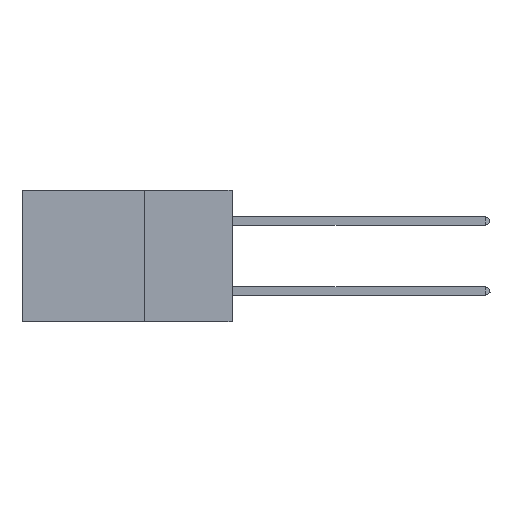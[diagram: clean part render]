
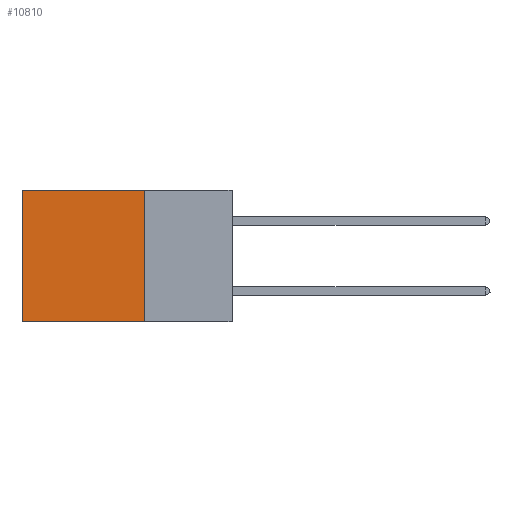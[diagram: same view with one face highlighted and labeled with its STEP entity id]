
A CAD part, left-side view. The second image highlights one B-rep face of the part: STEP entity #10810.
In plain terms, the highlighted planar face has unit normal (-1, 0, 0).
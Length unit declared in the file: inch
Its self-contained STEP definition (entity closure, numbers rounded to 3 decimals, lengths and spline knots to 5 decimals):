
#69 = VECTOR ( 'NONE', #7618, 39.37008 ) ;
#397 = DIRECTION ( 'NONE',  ( 0., 0., -1. ) ) ;
#1990 = DIRECTION ( 'NONE',  ( 0., 0., -1. ) ) ;
#3518 = VECTOR ( 'NONE', #1990, 39.37008 ) ;
#4175 = ORIENTED_EDGE ( 'NONE', *, *, #9058, .T. ) ;
#5876 = LINE ( 'NONE', #9888, #69 ) ;
#6025 = CARTESIAN_POINT ( 'NONE',  ( 0.2875, 0.25, -0.375 ) ) ;
#6129 = CARTESIAN_POINT ( 'NONE',  ( 0.2875, 0.6, -0.375 ) ) ;
#6674 = CARTESIAN_POINT ( 'NONE',  ( 0.2875, 0.25, -0.375 ) ) ;
#6875 = VERTEX_POINT ( 'NONE', #7212 ) ;
#6950 = VECTOR ( 'NONE', #9644, 39.37008 ) ;
#7188 = EDGE_CURVE ( 'NONE', #10684, #15488, #7501, .T. ) ;
#7212 = CARTESIAN_POINT ( 'NONE',  ( 0.2875, 0.6, -0.375 ) ) ;
#7288 = CARTESIAN_POINT ( 'NONE',  ( 0.2875, 0.25, 0. ) ) ;
#7501 = LINE ( 'NONE', #6674, #3518 ) ;
#7618 = DIRECTION ( 'NONE',  ( 0., 1., 0. ) ) ;
#7906 = EDGE_CURVE ( 'NONE', #11534, #6875, #13847, .T. ) ;
#9058 = EDGE_CURVE ( 'NONE', #10684, #11534, #11469, .T. ) ;
#9363 = VECTOR ( 'NONE', #13295, 39.37008 ) ;
#9644 = DIRECTION ( 'NONE',  ( 0., 1., 0. ) ) ;
#9843 = DIRECTION ( 'NONE',  ( 1., 0., 0. ) ) ;
#9888 = CARTESIAN_POINT ( 'NONE',  ( 0.2875, 0.25, -0.375 ) ) ;
#10684 = VERTEX_POINT ( 'NONE', #10763 ) ;
#10763 = CARTESIAN_POINT ( 'NONE',  ( 0.2875, 0.25, 0. ) ) ;
#10810 = ADVANCED_FACE ( 'NONE', ( #15540 ), #11066, .F. ) ;
#10960 = AXIS2_PLACEMENT_3D ( 'NONE', #13487, #9843, #397 ) ;
#11066 = PLANE ( 'NONE',  #10960 ) ;
#11469 = LINE ( 'NONE', #7288, #6950 ) ;
#11534 = VERTEX_POINT ( 'NONE', #14006 ) ;
#12342 = EDGE_CURVE ( 'NONE', #15488, #6875, #5876, .T. ) ;
#12413 = ORIENTED_EDGE ( 'NONE', *, *, #12342, .F. ) ;
#12878 = ORIENTED_EDGE ( 'NONE', *, *, #7906, .T. ) ;
#13113 = ORIENTED_EDGE ( 'NONE', *, *, #7188, .F. ) ;
#13295 = DIRECTION ( 'NONE',  ( 0., 0., -1. ) ) ;
#13487 = CARTESIAN_POINT ( 'NONE',  ( 0.2875, 0.25, -0.375 ) ) ;
#13847 = LINE ( 'NONE', #6129, #9363 ) ;
#14006 = CARTESIAN_POINT ( 'NONE',  ( 0.2875, 0.6, 0. ) ) ;
#14611 = EDGE_LOOP ( 'NONE', ( #12878, #12413, #13113, #4175 ) ) ;
#15488 = VERTEX_POINT ( 'NONE', #6025 ) ;
#15540 = FACE_OUTER_BOUND ( 'NONE', #14611, .T. ) ;
